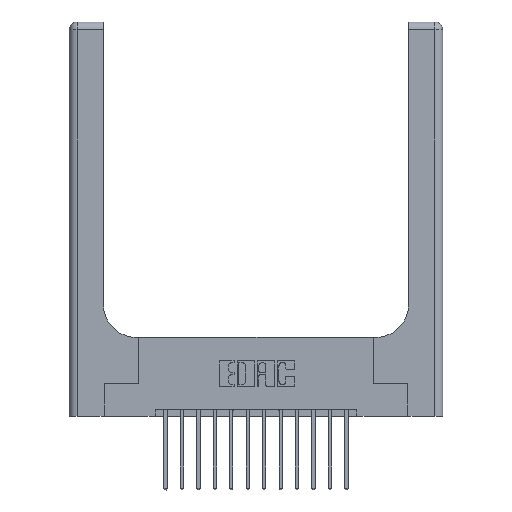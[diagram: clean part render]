
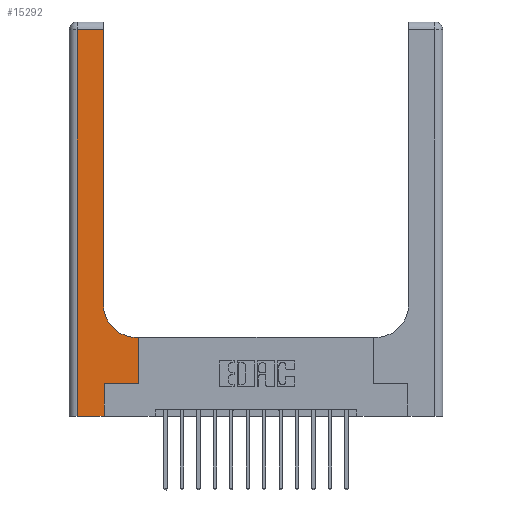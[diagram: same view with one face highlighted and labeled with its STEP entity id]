
A CAD part, top view. The second image highlights one B-rep face of the part: STEP entity #15292.
In plain terms, the highlighted planar face has unit normal (0, 0, 1).
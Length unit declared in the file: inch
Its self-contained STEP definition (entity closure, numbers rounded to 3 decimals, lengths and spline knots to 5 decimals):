
#4 = EDGE_CURVE ( 'NONE', #11815, #3131, #15670, .T. ) ;
#641 = DIRECTION ( 'NONE',  ( -1., 0., 0. ) ) ;
#1219 = DIRECTION ( 'NONE',  ( 1., 0., 0. ) ) ;
#1448 = EDGE_CURVE ( 'NONE', #6811, #7391, #9658, .T. ) ;
#1718 = DIRECTION ( 'NONE',  ( 1., 0., 0. ) ) ;
#1750 = LINE ( 'NONE', #13722, #14214 ) ;
#1765 = FACE_OUTER_BOUND ( 'NONE', #9788, .T. ) ;
#1855 = VECTOR ( 'NONE', #2246, 39.37008 ) ;
#2015 = VECTOR ( 'NONE', #4926, 39.37008 ) ;
#2246 = DIRECTION ( 'NONE',  ( 0., 1., 0. ) ) ;
#2273 = LINE ( 'NONE', #16613, #1855 ) ;
#2400 = EDGE_CURVE ( 'NONE', #16119, #10170, #7961, .T. ) ;
#2772 = CARTESIAN_POINT ( 'NONE',  ( 0.51, 0.6, 0.37 ) ) ;
#2846 = ORIENTED_EDGE ( 'NONE', *, *, #15931, .T. ) ;
#3008 = CARTESIAN_POINT ( 'NONE',  ( 0., 0., 0.37 ) ) ;
#3131 = VERTEX_POINT ( 'NONE', #12568 ) ;
#3205 = PLANE ( 'NONE',  #14797 ) ;
#3478 = DIRECTION ( 'NONE',  ( -1., 0., 0. ) ) ;
#3607 = CARTESIAN_POINT ( 'NONE',  ( 0.26, 0.6, 0.37 ) ) ;
#3646 = LINE ( 'NONE', #8514, #7998 ) ;
#3918 = CARTESIAN_POINT ( 'NONE',  ( 0.26, 0.85, 0.37 ) ) ;
#3975 = ORIENTED_EDGE ( 'NONE', *, *, #15399, .T. ) ;
#4315 = CARTESIAN_POINT ( 'NONE',  ( 0.26, 2.94, 0.37 ) ) ;
#4427 = VECTOR ( 'NONE', #15945, 39.37008 ) ;
#4926 = DIRECTION ( 'NONE',  ( -1., 0., 0. ) ) ;
#4966 = DIRECTION ( 'NONE',  ( 0., 1., 0. ) ) ;
#5035 = DIRECTION ( 'NONE',  ( 0., 0., -1. ) ) ;
#5738 = VERTEX_POINT ( 'NONE', #9151 ) ;
#5931 = CARTESIAN_POINT ( 'NONE',  ( 0.528, 0.6, 0.37 ) ) ;
#6231 = EDGE_CURVE ( 'NONE', #7391, #5738, #2273, .T. ) ;
#6811 = VERTEX_POINT ( 'NONE', #7555 ) ;
#6843 = CARTESIAN_POINT ( 'NONE',  ( 0.528, 0.25, 0.37 ) ) ;
#6938 = VECTOR ( 'NONE', #9436, 39.37008 ) ;
#7186 = VECTOR ( 'NONE', #3478, 39.37008 ) ;
#7391 = VERTEX_POINT ( 'NONE', #15608 ) ;
#7555 = CARTESIAN_POINT ( 'NONE',  ( 0.06, 0., 0.37 ) ) ;
#7651 = ORIENTED_EDGE ( 'NONE', *, *, #2400, .T. ) ;
#7819 = LINE ( 'NONE', #3607, #7186 ) ;
#7826 = VERTEX_POINT ( 'NONE', #3918 ) ;
#7961 = LINE ( 'NONE', #6843, #4427 ) ;
#7998 = VECTOR ( 'NONE', #16201, 39.37008 ) ;
#8040 = EDGE_CURVE ( 'NONE', #10170, #15742, #7819, .T. ) ;
#8514 = CARTESIAN_POINT ( 'NONE',  ( 0.06, 3., 0.37 ) ) ;
#8940 = AXIS2_PLACEMENT_3D ( 'NONE', #11654, #5035, #1219 ) ;
#9151 = CARTESIAN_POINT ( 'NONE',  ( 0.265, 0.25, 0.37 ) ) ;
#9436 = DIRECTION ( 'NONE',  ( 1., 0., 0. ) ) ;
#9651 = VECTOR ( 'NONE', #4966, 39.37008 ) ;
#9658 = LINE ( 'NONE', #3008, #6938 ) ;
#9788 = EDGE_LOOP ( 'NONE', ( #13676, #10622, #3975, #15457, #11702, #2846, #7651, #12015, #12510 ) ) ;
#9896 = CARTESIAN_POINT ( 'NONE',  ( 0., 3., 0.37 ) ) ;
#10170 = VERTEX_POINT ( 'NONE', #5931 ) ;
#10622 = ORIENTED_EDGE ( 'NONE', *, *, #4, .T. ) ;
#11416 = CARTESIAN_POINT ( 'NONE',  ( 0.528, 0.25, 0.37 ) ) ;
#11581 = CARTESIAN_POINT ( 'NONE',  ( 0.26, 3., 0.37 ) ) ;
#11654 = CARTESIAN_POINT ( 'NONE',  ( 0.51, 0.85, 0.37 ) ) ;
#11702 = ORIENTED_EDGE ( 'NONE', *, *, #6231, .T. ) ;
#11815 = VERTEX_POINT ( 'NONE', #4315 ) ;
#12015 = ORIENTED_EDGE ( 'NONE', *, *, #8040, .T. ) ;
#12304 = LINE ( 'NONE', #11581, #9651 ) ;
#12510 = ORIENTED_EDGE ( 'NONE', *, *, #13417, .T. ) ;
#12568 = CARTESIAN_POINT ( 'NONE',  ( 0.06, 2.94, 0.37 ) ) ;
#13251 = CIRCLE ( 'NONE', #8940, 0.25 ) ;
#13417 = EDGE_CURVE ( 'NONE', #15742, #7826, #13251, .T. ) ;
#13654 = DIRECTION ( 'NONE',  ( 0., 0., -1. ) ) ;
#13676 = ORIENTED_EDGE ( 'NONE', *, *, #16295, .T. ) ;
#13722 = CARTESIAN_POINT ( 'NONE',  ( 0.265, 0.25, 0.37 ) ) ;
#14098 = CARTESIAN_POINT ( 'NONE',  ( 0., 2.94, 0.37 ) ) ;
#14214 = VECTOR ( 'NONE', #1718, 39.37008 ) ;
#14797 = AXIS2_PLACEMENT_3D ( 'NONE', #9896, #13654, #641 ) ;
#15292 = ADVANCED_FACE ( 'NONE', ( #1765 ), #3205, .F. ) ;
#15399 = EDGE_CURVE ( 'NONE', #3131, #6811, #3646, .T. ) ;
#15457 = ORIENTED_EDGE ( 'NONE', *, *, #1448, .T. ) ;
#15608 = CARTESIAN_POINT ( 'NONE',  ( 0.265, 0., 0.37 ) ) ;
#15670 = LINE ( 'NONE', #14098, #2015 ) ;
#15742 = VERTEX_POINT ( 'NONE', #2772 ) ;
#15931 = EDGE_CURVE ( 'NONE', #5738, #16119, #1750, .T. ) ;
#15945 = DIRECTION ( 'NONE',  ( 0., 1., 0. ) ) ;
#16119 = VERTEX_POINT ( 'NONE', #11416 ) ;
#16201 = DIRECTION ( 'NONE',  ( 0., -1., 0. ) ) ;
#16295 = EDGE_CURVE ( 'NONE', #7826, #11815, #12304, .T. ) ;
#16613 = CARTESIAN_POINT ( 'NONE',  ( 0.265, 0., 0.37 ) ) ;
